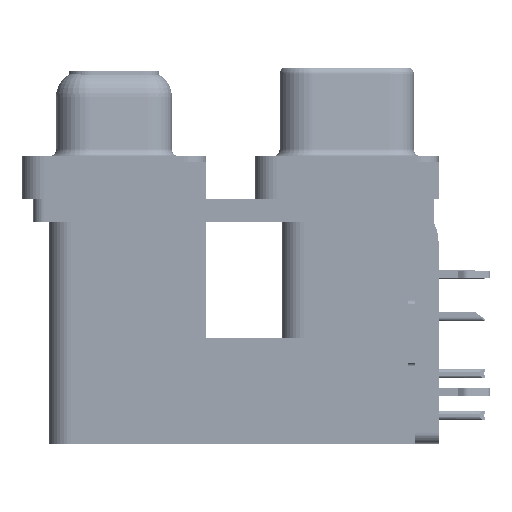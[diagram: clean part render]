
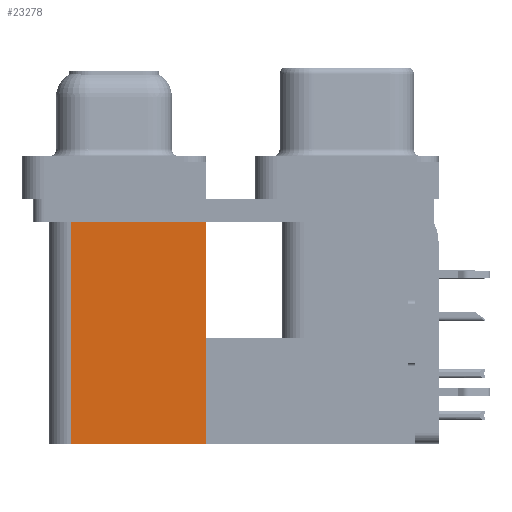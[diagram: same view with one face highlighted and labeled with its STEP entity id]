
A CAD part, left-side view. The second image highlights one B-rep face of the part: STEP entity #23278.
In plain terms, the highlighted planar face has unit normal (-1, 0, 0).
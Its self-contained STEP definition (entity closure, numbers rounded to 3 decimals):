
#715 = DIRECTION ( 'NONE',  ( 0., 1., 0. ) ) ;
#1295 = CARTESIAN_POINT ( 'NONE',  ( 3.7, 9.6, -19.2 ) ) ;
#2422 = CARTESIAN_POINT ( 'NONE',  ( 3.7, 9.6, -2.5 ) ) ;
#6736 = FACE_OUTER_BOUND ( 'NONE', #21196, .T. ) ;
#6814 = ORIENTED_EDGE ( 'NONE', *, *, #37337, .F. ) ;
#8386 = DIRECTION ( 'NONE',  ( 0., 1., 0. ) ) ;
#10049 = AXIS2_PLACEMENT_3D ( 'NONE', #29144, #51542, #20427 ) ;
#11383 = PLANE ( 'NONE',  #10049 ) ;
#13183 = EDGE_CURVE ( 'NONE', #28836, #51570, #22262, .T. ) ;
#13196 = EDGE_CURVE ( 'NONE', #49897, #28836, #18470, .T. ) ;
#13805 = DIRECTION ( 'NONE',  ( 0., 0., 1. ) ) ;
#14084 = CARTESIAN_POINT ( 'NONE',  ( 3.7, 9.6, -2.5 ) ) ;
#14879 = CARTESIAN_POINT ( 'NONE',  ( 3.7, 18.8, -19.2 ) ) ;
#16143 = ORIENTED_EDGE ( 'NONE', *, *, #46116, .F. ) ;
#17426 = CARTESIAN_POINT ( 'NONE',  ( 3.7, 9.6, -19.2 ) ) ;
#18470 = LINE ( 'NONE', #1295, #22567 ) ;
#20427 = DIRECTION ( 'NONE',  ( 0., 0., -1. ) ) ;
#21196 = EDGE_LOOP ( 'NONE', ( #23843, #6814, #16143, #33794 ) ) ;
#22262 = LINE ( 'NONE', #14084, #50460 ) ;
#22567 = VECTOR ( 'NONE', #13805, 1000. ) ;
#23278 = ADVANCED_FACE ( 'NONE', ( #6736 ), #11383, .F. ) ;
#23603 = CARTESIAN_POINT ( 'NONE',  ( 3.7, 18.8, -2.5 ) ) ;
#23843 = ORIENTED_EDGE ( 'NONE', *, *, #13183, .T. ) ;
#28836 = VERTEX_POINT ( 'NONE', #2422 ) ;
#28963 = CARTESIAN_POINT ( 'NONE',  ( 3.7, 18.8, -19.2 ) ) ;
#29144 = CARTESIAN_POINT ( 'NONE',  ( 3.7, 9.6, -19.2 ) ) ;
#32631 = DIRECTION ( 'NONE',  ( 0., 0., 1. ) ) ;
#33504 = VERTEX_POINT ( 'NONE', #28963 ) ;
#33794 = ORIENTED_EDGE ( 'NONE', *, *, #13196, .T. ) ;
#35446 = LINE ( 'NONE', #17426, #38715 ) ;
#37337 = EDGE_CURVE ( 'NONE', #33504, #51570, #44856, .T. ) ;
#38715 = VECTOR ( 'NONE', #8386, 1000. ) ;
#40006 = VECTOR ( 'NONE', #32631, 1000. ) ;
#44856 = LINE ( 'NONE', #14879, #40006 ) ;
#46116 = EDGE_CURVE ( 'NONE', #49897, #33504, #35446, .T. ) ;
#49897 = VERTEX_POINT ( 'NONE', #50376 ) ;
#50376 = CARTESIAN_POINT ( 'NONE',  ( 3.7, 9.6, -19.2 ) ) ;
#50460 = VECTOR ( 'NONE', #715, 1000. ) ;
#51542 = DIRECTION ( 'NONE',  ( 1., 0., 0. ) ) ;
#51570 = VERTEX_POINT ( 'NONE', #23603 ) ;
